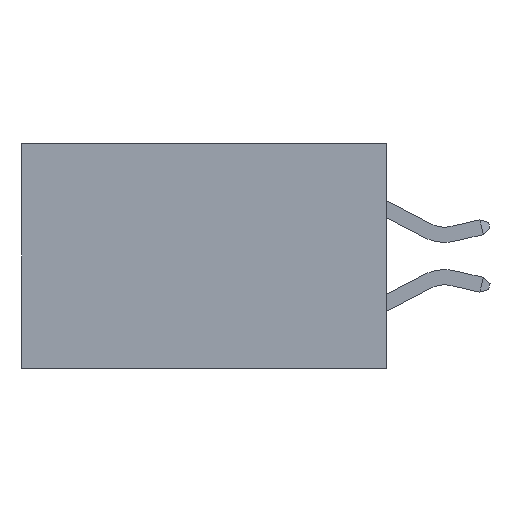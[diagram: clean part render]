
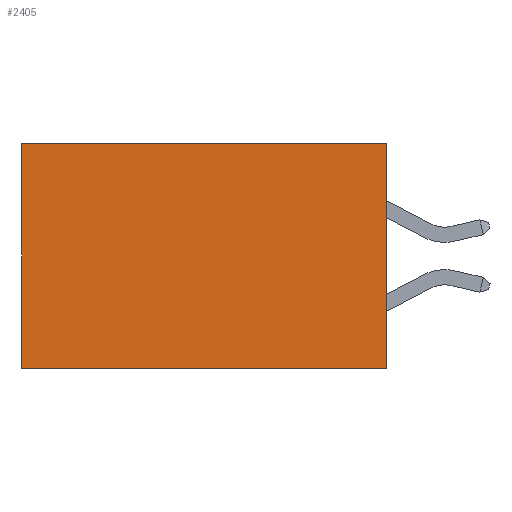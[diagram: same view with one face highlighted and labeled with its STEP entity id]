
A CAD part, left-side view. The second image highlights one B-rep face of the part: STEP entity #2405.
In plain terms, the highlighted planar face has unit normal (-1, 0, 0).
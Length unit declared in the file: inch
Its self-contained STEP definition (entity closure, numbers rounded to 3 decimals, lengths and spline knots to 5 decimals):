
#1258 = VECTOR ( 'NONE', #13627, 39.37008 ) ;
#2169 = AXIS2_PLACEMENT_3D ( 'NONE', #27670, #12891, #2650 ) ;
#2405 = ADVANCED_FACE ( 'NONE', ( #15436 ), #5262, .F. ) ;
#2650 = DIRECTION ( 'NONE',  ( 0., 0., -1. ) ) ;
#2948 = CARTESIAN_POINT ( 'NONE',  ( 0.298, 0.6, 0. ) ) ;
#3165 = CARTESIAN_POINT ( 'NONE',  ( 0.298, 0., 0. ) ) ;
#3816 = EDGE_CURVE ( 'NONE', #31132, #4014, #12256, .T. ) ;
#4014 = VERTEX_POINT ( 'NONE', #30827 ) ;
#5120 = VECTOR ( 'NONE', #28374, 39.37008 ) ;
#5262 = PLANE ( 'NONE',  #2169 ) ;
#7893 = DIRECTION ( 'NONE',  ( 0., 0., -1. ) ) ;
#7954 = LINE ( 'NONE', #2948, #31507 ) ;
#9697 = VECTOR ( 'NONE', #15688, 39.37008 ) ;
#10566 = CARTESIAN_POINT ( 'NONE',  ( 0.298, 0., 0. ) ) ;
#12256 = LINE ( 'NONE', #20563, #5120 ) ;
#12891 = DIRECTION ( 'NONE',  ( 1., 0., 0. ) ) ;
#13627 = DIRECTION ( 'NONE',  ( 0., 0., -1. ) ) ;
#13765 = VERTEX_POINT ( 'NONE', #25864 ) ;
#14401 = LINE ( 'NONE', #17985, #9697 ) ;
#14616 = LINE ( 'NONE', #3165, #1258 ) ;
#15436 = FACE_OUTER_BOUND ( 'NONE', #21789, .T. ) ;
#15688 = DIRECTION ( 'NONE',  ( 0., 1., 0. ) ) ;
#17985 = CARTESIAN_POINT ( 'NONE',  ( 0.298, 0., 0. ) ) ;
#18815 = ORIENTED_EDGE ( 'NONE', *, *, #25703, .F. ) ;
#18906 = ORIENTED_EDGE ( 'NONE', *, *, #3816, .F. ) ;
#18943 = EDGE_CURVE ( 'NONE', #13765, #4014, #7954, .T. ) ;
#20085 = VERTEX_POINT ( 'NONE', #10566 ) ;
#20563 = CARTESIAN_POINT ( 'NONE',  ( 0.298, 0., -0.37 ) ) ;
#21789 = EDGE_LOOP ( 'NONE', ( #32108, #18906, #18815, #28151 ) ) ;
#23048 = EDGE_CURVE ( 'NONE', #20085, #13765, #14401, .T. ) ;
#25703 = EDGE_CURVE ( 'NONE', #20085, #31132, #14616, .T. ) ;
#25864 = CARTESIAN_POINT ( 'NONE',  ( 0.298, 0.6, 0. ) ) ;
#27637 = CARTESIAN_POINT ( 'NONE',  ( 0.298, 0., -0.37 ) ) ;
#27670 = CARTESIAN_POINT ( 'NONE',  ( 0.298, 0., 0. ) ) ;
#28151 = ORIENTED_EDGE ( 'NONE', *, *, #23048, .T. ) ;
#28374 = DIRECTION ( 'NONE',  ( 0., 1., 0. ) ) ;
#30827 = CARTESIAN_POINT ( 'NONE',  ( 0.298, 0.6, -0.37 ) ) ;
#31132 = VERTEX_POINT ( 'NONE', #27637 ) ;
#31507 = VECTOR ( 'NONE', #7893, 39.37008 ) ;
#32108 = ORIENTED_EDGE ( 'NONE', *, *, #18943, .T. ) ;
